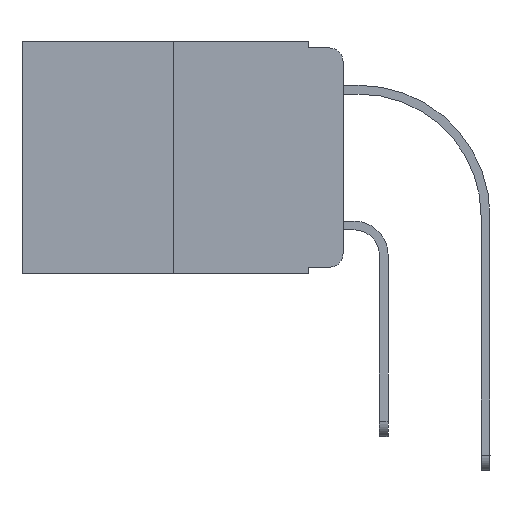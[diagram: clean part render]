
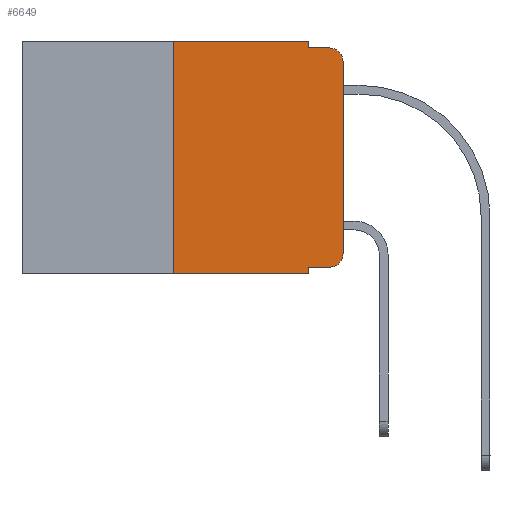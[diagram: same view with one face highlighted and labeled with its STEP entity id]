
A CAD part, left-side view. The second image highlights one B-rep face of the part: STEP entity #6649.
In plain terms, the highlighted planar face has unit normal (-1, 0, 0).
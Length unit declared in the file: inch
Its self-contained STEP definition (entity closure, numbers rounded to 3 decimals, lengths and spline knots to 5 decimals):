
#238 = CARTESIAN_POINT ( 'NONE',  ( 0., 0.473, -0.343 ) ) ;
#721 = VERTEX_POINT ( 'NONE', #12581 ) ;
#1690 = VERTEX_POINT ( 'NONE', #23638 ) ;
#2034 = VERTEX_POINT ( 'NONE', #24897 ) ;
#2243 = EDGE_CURVE ( 'NONE', #1690, #721, #2792, .T. ) ;
#2792 = LINE ( 'NONE', #24838, #23918 ) ;
#2865 = CARTESIAN_POINT ( 'NONE',  ( 0., 0.473, 0. ) ) ;
#3212 = ORIENTED_EDGE ( 'NONE', *, *, #22114, .T. ) ;
#3716 = VECTOR ( 'NONE', #22715, 39.37008 ) ;
#4281 = VERTEX_POINT ( 'NONE', #14384 ) ;
#4591 = DIRECTION ( 'NONE',  ( 0., -1., 0. ) ) ;
#4801 = PLANE ( 'NONE',  #7854 ) ;
#5100 = LINE ( 'NONE', #8709, #24079 ) ;
#5185 = DIRECTION ( 'NONE',  ( 0., 0., 1. ) ) ;
#5409 = CARTESIAN_POINT ( 'NONE',  ( 0., 0.051, -0.01 ) ) ;
#5794 = CIRCLE ( 'NONE', #16089, 0.02 ) ;
#5892 = DIRECTION ( 'NONE',  ( 0., -1., 0. ) ) ;
#5909 = VERTEX_POINT ( 'NONE', #12211 ) ;
#6611 = EDGE_CURVE ( 'NONE', #2034, #23054, #12785, .T. ) ;
#6649 = ADVANCED_FACE ( 'NONE', ( #22958 ), #4801, .F. ) ;
#7133 = CARTESIAN_POINT ( 'NONE',  ( 0., 0., 0. ) ) ;
#7348 = VECTOR ( 'NONE', #17957, 39.37008 ) ;
#7739 = AXIS2_PLACEMENT_3D ( 'NONE', #25097, #19179, #11565 ) ;
#7854 = AXIS2_PLACEMENT_3D ( 'NONE', #2865, #8805, #16664 ) ;
#7974 = LINE ( 'NONE', #238, #15587 ) ;
#8709 = CARTESIAN_POINT ( 'NONE',  ( 0., 0.051, 0. ) ) ;
#8805 = DIRECTION ( 'NONE',  ( 1., 0., 0. ) ) ;
#9455 = CARTESIAN_POINT ( 'NONE',  ( 0., 0.051, -0.333 ) ) ;
#9504 = LINE ( 'NONE', #17377, #13196 ) ;
#10419 = VERTEX_POINT ( 'NONE', #9455 ) ;
#10573 = ORIENTED_EDGE ( 'NONE', *, *, #14105, .F. ) ;
#10765 = EDGE_CURVE ( 'NONE', #5909, #1690, #22840, .T. ) ;
#11565 = DIRECTION ( 'NONE',  ( 0., 0., -1. ) ) ;
#11965 = VERTEX_POINT ( 'NONE', #25316 ) ;
#12166 = VERTEX_POINT ( 'NONE', #20399 ) ;
#12211 = CARTESIAN_POINT ( 'NONE',  ( 0., 0.25, -0.343 ) ) ;
#12581 = CARTESIAN_POINT ( 'NONE',  ( 0., 0.051, 0. ) ) ;
#12785 = LINE ( 'NONE', #7133, #3716 ) ;
#13196 = VECTOR ( 'NONE', #5892, 39.37008 ) ;
#14105 = EDGE_CURVE ( 'NONE', #18022, #11965, #23196, .T. ) ;
#14384 = CARTESIAN_POINT ( 'NONE',  ( 0., 0.02, -0.333 ) ) ;
#14714 = ORIENTED_EDGE ( 'NONE', *, *, #14747, .F. ) ;
#14747 = EDGE_CURVE ( 'NONE', #721, #18022, #5100, .T. ) ;
#15587 = VECTOR ( 'NONE', #4591, 39.37008 ) ;
#15709 = DIRECTION ( 'NONE',  ( 0., -1., 0. ) ) ;
#15825 = VECTOR ( 'NONE', #15709, 39.37008 ) ;
#16089 = AXIS2_PLACEMENT_3D ( 'NONE', #23681, #19431, #21741 ) ;
#16664 = DIRECTION ( 'NONE',  ( 0., 0., -1. ) ) ;
#16783 = CARTESIAN_POINT ( 'NONE',  ( 0., 0.25, 0. ) ) ;
#16889 = CARTESIAN_POINT ( 'NONE',  ( 0., 0., -0.03 ) ) ;
#16928 = EDGE_CURVE ( 'NONE', #5909, #12166, #7974, .T. ) ;
#17105 = DIRECTION ( 'NONE',  ( 0., -1., 0. ) ) ;
#17365 = VECTOR ( 'NONE', #5185, 39.37008 ) ;
#17377 = CARTESIAN_POINT ( 'NONE',  ( 0., 0.051, -0.333 ) ) ;
#17957 = DIRECTION ( 'NONE',  ( 0., 0., -1. ) ) ;
#18022 = VERTEX_POINT ( 'NONE', #22663 ) ;
#19179 = DIRECTION ( 'NONE',  ( -1., 0., 0. ) ) ;
#19431 = DIRECTION ( 'NONE',  ( -1., 0., 0. ) ) ;
#19675 = CIRCLE ( 'NONE', #7739, 0.02 ) ;
#20253 = LINE ( 'NONE', #21815, #7348 ) ;
#20399 = CARTESIAN_POINT ( 'NONE',  ( 0., 0.051, -0.343 ) ) ;
#20455 = EDGE_CURVE ( 'NONE', #4281, #2034, #5794, .T. ) ;
#20524 = EDGE_CURVE ( 'NONE', #10419, #4281, #9504, .T. ) ;
#20552 = DIRECTION ( 'NONE',  ( 0., 0., -1. ) ) ;
#20721 = ORIENTED_EDGE ( 'NONE', *, *, #16928, .T. ) ;
#21177 = ORIENTED_EDGE ( 'NONE', *, *, #2243, .F. ) ;
#21741 = DIRECTION ( 'NONE',  ( 0., 0., -1. ) ) ;
#21815 = CARTESIAN_POINT ( 'NONE',  ( 0., 0.051, 0. ) ) ;
#22114 = EDGE_CURVE ( 'NONE', #23054, #11965, #19675, .T. ) ;
#22275 = ORIENTED_EDGE ( 'NONE', *, *, #20524, .T. ) ;
#22663 = CARTESIAN_POINT ( 'NONE',  ( 0., 0.051, -0.01 ) ) ;
#22715 = DIRECTION ( 'NONE',  ( 0., 0., 1. ) ) ;
#22840 = LINE ( 'NONE', #16783, #17365 ) ;
#22857 = EDGE_CURVE ( 'NONE', #10419, #12166, #20253, .T. ) ;
#22958 = FACE_OUTER_BOUND ( 'NONE', #24398, .T. ) ;
#23054 = VERTEX_POINT ( 'NONE', #16889 ) ;
#23196 = LINE ( 'NONE', #5409, #15825 ) ;
#23638 = CARTESIAN_POINT ( 'NONE',  ( 0., 0.25, 0. ) ) ;
#23681 = CARTESIAN_POINT ( 'NONE',  ( 0., 0.02, -0.313 ) ) ;
#23918 = VECTOR ( 'NONE', #17105, 39.37008 ) ;
#24079 = VECTOR ( 'NONE', #20552, 39.37008 ) ;
#24134 = ORIENTED_EDGE ( 'NONE', *, *, #10765, .F. ) ;
#24398 = EDGE_LOOP ( 'NONE', ( #24498, #3212, #10573, #14714, #21177, #24134, #20721, #25089, #22275, #24987 ) ) ;
#24498 = ORIENTED_EDGE ( 'NONE', *, *, #6611, .T. ) ;
#24838 = CARTESIAN_POINT ( 'NONE',  ( 0., 0.473, 0. ) ) ;
#24897 = CARTESIAN_POINT ( 'NONE',  ( 0., 0., -0.313 ) ) ;
#24987 = ORIENTED_EDGE ( 'NONE', *, *, #20455, .T. ) ;
#25089 = ORIENTED_EDGE ( 'NONE', *, *, #22857, .F. ) ;
#25097 = CARTESIAN_POINT ( 'NONE',  ( 0., 0.02, -0.03 ) ) ;
#25316 = CARTESIAN_POINT ( 'NONE',  ( 0., 0.02, -0.01 ) ) ;
